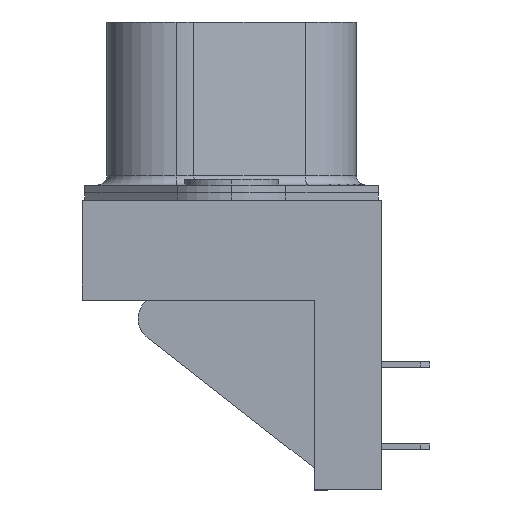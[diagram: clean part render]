
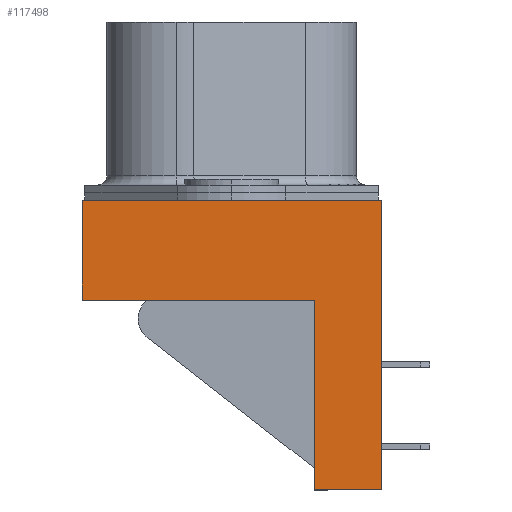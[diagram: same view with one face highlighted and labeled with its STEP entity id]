
A CAD part, left-side view. The second image highlights one B-rep face of the part: STEP entity #117498.
In plain terms, the highlighted planar face has unit normal (-1, 0, 0).
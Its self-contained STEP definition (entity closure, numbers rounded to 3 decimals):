
#11675 = VECTOR ( 'NONE', #139921, 1000. ) ;
#12178 = DIRECTION ( 'NONE',  ( 0., -1., 0. ) ) ;
#13127 = VERTEX_POINT ( 'NONE', #38891 ) ;
#13490 = ORIENTED_EDGE ( 'NONE', *, *, #154051, .F. ) ;
#18025 = CARTESIAN_POINT ( 'NONE',  ( -4.125, 7.8, 0. ) ) ;
#19869 = ORIENTED_EDGE ( 'NONE', *, *, #63563, .F. ) ;
#21414 = LINE ( 'NONE', #50465, #114211 ) ;
#25817 = FACE_OUTER_BOUND ( 'NONE', #37490, .T. ) ;
#26817 = CARTESIAN_POINT ( 'NONE',  ( -4.125, -4.3, -15.1 ) ) ;
#34698 = CARTESIAN_POINT ( 'NONE',  ( -4.125, -4.3, -5.2 ) ) ;
#35368 = DIRECTION ( 'NONE',  ( 0., 1., 0. ) ) ;
#37490 = EDGE_LOOP ( 'NONE', ( #127717, #19869, #143137, #83786, #13490, #161607 ) ) ;
#38891 = CARTESIAN_POINT ( 'NONE',  ( -4.125, 7.8, -5.2 ) ) ;
#39237 = AXIS2_PLACEMENT_3D ( 'NONE', #162320, #136828, #12178 ) ;
#43293 = VERTEX_POINT ( 'NONE', #18025 ) ;
#50439 = VERTEX_POINT ( 'NONE', #151524 ) ;
#50465 = CARTESIAN_POINT ( 'NONE',  ( -4.125, -7.8, -15.1 ) ) ;
#50976 = VECTOR ( 'NONE', #129212, 1000. ) ;
#55128 = LINE ( 'NONE', #166128, #145561 ) ;
#56806 = DIRECTION ( 'NONE',  ( 0., 0., 1. ) ) ;
#58906 = CARTESIAN_POINT ( 'NONE',  ( -4.125, 7.8, -15.1 ) ) ;
#62372 = DIRECTION ( 'NONE',  ( 0., 0., 1. ) ) ;
#63563 = EDGE_CURVE ( 'NONE', #175952, #85089, #70476, .T. ) ;
#66170 = EDGE_CURVE ( 'NONE', #50439, #116253, #21414, .T. ) ;
#70476 = LINE ( 'NONE', #26817, #107666 ) ;
#73693 = CARTESIAN_POINT ( 'NONE',  ( -4.125, 7.8, -15.1 ) ) ;
#83786 = ORIENTED_EDGE ( 'NONE', *, *, #66170, .T. ) ;
#84422 = LINE ( 'NONE', #58906, #11675 ) ;
#85089 = VERTEX_POINT ( 'NONE', #34698 ) ;
#86613 = EDGE_CURVE ( 'NONE', #175952, #50439, #90030, .T. ) ;
#90030 = LINE ( 'NONE', #73693, #50976 ) ;
#95196 = DIRECTION ( 'NONE',  ( 0., -1., 0. ) ) ;
#99121 = CARTESIAN_POINT ( 'NONE',  ( -4.125, 7.8, -5.2 ) ) ;
#106813 = PLANE ( 'NONE',  #39237 ) ;
#107666 = VECTOR ( 'NONE', #56806, 1000. ) ;
#111053 = EDGE_CURVE ( 'NONE', #85089, #13127, #126468, .T. ) ;
#114211 = VECTOR ( 'NONE', #62372, 1000. ) ;
#116253 = VERTEX_POINT ( 'NONE', #171367 ) ;
#117498 = ADVANCED_FACE ( 'NONE', ( #25817 ), #106813, .T. ) ;
#126468 = LINE ( 'NONE', #99121, #150476 ) ;
#127717 = ORIENTED_EDGE ( 'NONE', *, *, #111053, .F. ) ;
#129212 = DIRECTION ( 'NONE',  ( 0., -1., 0. ) ) ;
#136828 = DIRECTION ( 'NONE',  ( -1., 0., 0. ) ) ;
#139921 = DIRECTION ( 'NONE',  ( 0., 0., 1. ) ) ;
#143137 = ORIENTED_EDGE ( 'NONE', *, *, #86613, .T. ) ;
#145561 = VECTOR ( 'NONE', #95196, 1000. ) ;
#147229 = EDGE_CURVE ( 'NONE', #13127, #43293, #84422, .T. ) ;
#148392 = CARTESIAN_POINT ( 'NONE',  ( -4.125, -4.3, -15.1 ) ) ;
#150476 = VECTOR ( 'NONE', #35368, 1000. ) ;
#151524 = CARTESIAN_POINT ( 'NONE',  ( -4.125, -7.8, -15.1 ) ) ;
#154051 = EDGE_CURVE ( 'NONE', #43293, #116253, #55128, .T. ) ;
#161607 = ORIENTED_EDGE ( 'NONE', *, *, #147229, .F. ) ;
#162320 = CARTESIAN_POINT ( 'NONE',  ( -4.125, 7.8, -15.1 ) ) ;
#166128 = CARTESIAN_POINT ( 'NONE',  ( -4.125, 7.8, 0. ) ) ;
#171367 = CARTESIAN_POINT ( 'NONE',  ( -4.125, -7.8, 0. ) ) ;
#175952 = VERTEX_POINT ( 'NONE', #148392 ) ;
